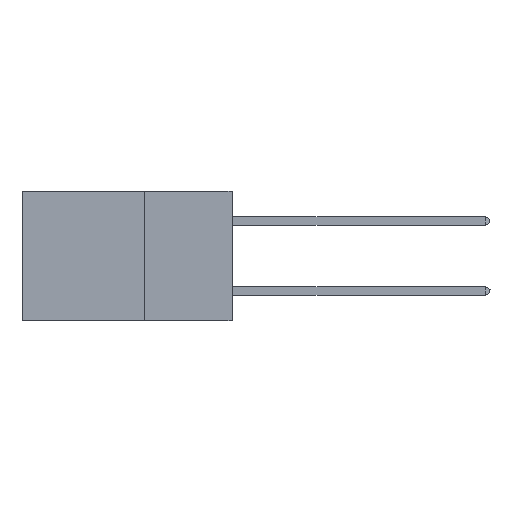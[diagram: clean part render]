
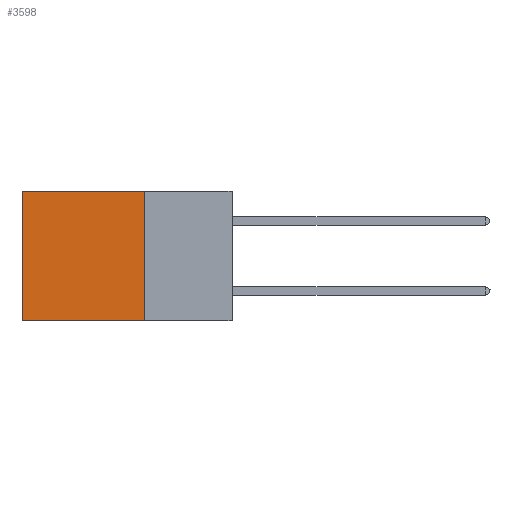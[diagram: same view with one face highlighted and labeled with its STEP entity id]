
A CAD part, left-side view. The second image highlights one B-rep face of the part: STEP entity #3598.
In plain terms, the highlighted planar face has unit normal (-1, 0, 0).
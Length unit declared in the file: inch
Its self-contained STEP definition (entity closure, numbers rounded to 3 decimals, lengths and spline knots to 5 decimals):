
#498 = LINE ( 'NONE', #28299, #29898 ) ;
#1519 = DIRECTION ( 'NONE',  ( 0., 1., 0. ) ) ;
#1546 = LINE ( 'NONE', #23168, #30071 ) ;
#1687 = EDGE_CURVE ( 'NONE', #19596, #17529, #10862, .T. ) ;
#3598 = ADVANCED_FACE ( 'NONE', ( #18162 ), #14663, .F. ) ;
#4719 = EDGE_CURVE ( 'NONE', #19596, #29853, #5940, .T. ) ;
#5940 = LINE ( 'NONE', #10152, #28752 ) ;
#8244 = DIRECTION ( 'NONE',  ( 0., 0., -1. ) ) ;
#9962 = DIRECTION ( 'NONE',  ( 1., 0., 0. ) ) ;
#10152 = CARTESIAN_POINT ( 'NONE',  ( 0.2875, 0.25, 0. ) ) ;
#10497 = CARTESIAN_POINT ( 'NONE',  ( 0.2875, 0.25, 0. ) ) ;
#10862 = LINE ( 'NONE', #15968, #32653 ) ;
#11839 = EDGE_LOOP ( 'NONE', ( #16642, #21217, #17019, #35401 ) ) ;
#12356 = CARTESIAN_POINT ( 'NONE',  ( 0.2875, 0.6, -0.37 ) ) ;
#14663 = PLANE ( 'NONE',  #29079 ) ;
#15968 = CARTESIAN_POINT ( 'NONE',  ( 0.2875, 0.25, 0. ) ) ;
#16642 = ORIENTED_EDGE ( 'NONE', *, *, #36576, .T. ) ;
#17019 = ORIENTED_EDGE ( 'NONE', *, *, #4719, .F. ) ;
#17529 = VERTEX_POINT ( 'NONE', #21775 ) ;
#17683 = DIRECTION ( 'NONE',  ( 0., 0., -1. ) ) ;
#18162 = FACE_OUTER_BOUND ( 'NONE', #11839, .T. ) ;
#19596 = VERTEX_POINT ( 'NONE', #10497 ) ;
#21217 = ORIENTED_EDGE ( 'NONE', *, *, #23465, .F. ) ;
#21296 = CARTESIAN_POINT ( 'NONE',  ( 0.2875, 0.25, 0. ) ) ;
#21369 = CARTESIAN_POINT ( 'NONE',  ( 0.2875, 0.25, -0.37 ) ) ;
#21775 = CARTESIAN_POINT ( 'NONE',  ( 0.2875, 0.6, 0. ) ) ;
#23168 = CARTESIAN_POINT ( 'NONE',  ( 0.2875, 0.25, -0.37 ) ) ;
#23465 = EDGE_CURVE ( 'NONE', #29853, #28566, #1546, .T. ) ;
#28187 = DIRECTION ( 'NONE',  ( 0., 0., -1. ) ) ;
#28299 = CARTESIAN_POINT ( 'NONE',  ( 0.2875, 0.6, 0. ) ) ;
#28566 = VERTEX_POINT ( 'NONE', #12356 ) ;
#28752 = VECTOR ( 'NONE', #8244, 39.37008 ) ;
#29079 = AXIS2_PLACEMENT_3D ( 'NONE', #21296, #9962, #17683 ) ;
#29853 = VERTEX_POINT ( 'NONE', #21369 ) ;
#29898 = VECTOR ( 'NONE', #28187, 39.37008 ) ;
#30071 = VECTOR ( 'NONE', #31363, 39.37008 ) ;
#31363 = DIRECTION ( 'NONE',  ( 0., 1., 0. ) ) ;
#32653 = VECTOR ( 'NONE', #1519, 39.37008 ) ;
#35401 = ORIENTED_EDGE ( 'NONE', *, *, #1687, .T. ) ;
#36576 = EDGE_CURVE ( 'NONE', #17529, #28566, #498, .T. ) ;
